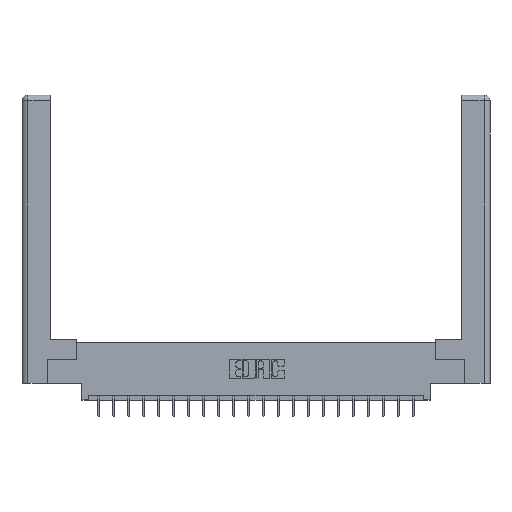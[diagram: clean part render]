
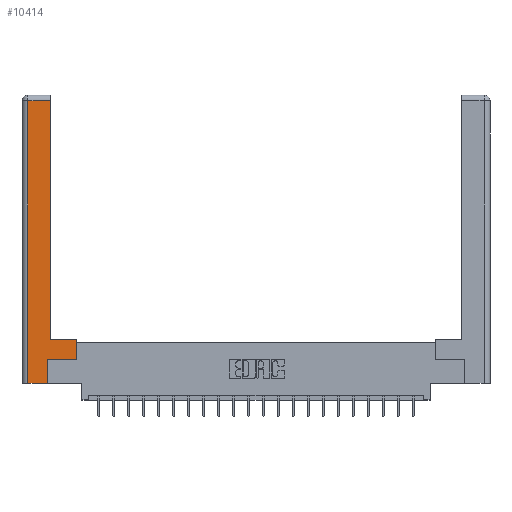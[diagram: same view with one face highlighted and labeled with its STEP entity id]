
A CAD part, top view. The second image highlights one B-rep face of the part: STEP entity #10414.
In plain terms, the highlighted planar face has unit normal (0, 0, 1).
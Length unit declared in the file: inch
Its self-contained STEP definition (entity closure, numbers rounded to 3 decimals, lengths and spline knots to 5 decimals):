
#24 = FACE_OUTER_BOUND ( 'NONE', #19741, .T. ) ;
#35 = LINE ( 'NONE', #14683, #7109 ) ;
#592 = CARTESIAN_POINT ( 'NONE',  ( 0.565, 0.245, 0. ) ) ;
#648 = DIRECTION ( 'NONE',  ( -1., 0., 0. ) ) ;
#887 = CARTESIAN_POINT ( 'NONE',  ( 0.0615, 2.94, 0. ) ) ;
#1226 = LINE ( 'NONE', #21098, #18644 ) ;
#1775 = VERTEX_POINT ( 'NONE', #4766 ) ;
#2141 = EDGE_CURVE ( 'NONE', #1775, #12506, #17856, .T. ) ;
#2516 = VECTOR ( 'NONE', #10026, 39.37008 ) ;
#2885 = EDGE_CURVE ( 'NONE', #7992, #18222, #19968, .T. ) ;
#3042 = EDGE_CURVE ( 'NONE', #20819, #6020, #1226, .T. ) ;
#4004 = DIRECTION ( 'NONE',  ( -1., 0., 0. ) ) ;
#4051 = CARTESIAN_POINT ( 'NONE',  ( 0.0615, 0., 0. ) ) ;
#4662 = AXIS2_PLACEMENT_3D ( 'NONE', #17757, #10466, #12505 ) ;
#4766 = CARTESIAN_POINT ( 'NONE',  ( 0.565, 0.45, 0. ) ) ;
#4906 = ORIENTED_EDGE ( 'NONE', *, *, #7469, .T. ) ;
#5986 = ORIENTED_EDGE ( 'NONE', *, *, #10708, .T. ) ;
#6020 = VERTEX_POINT ( 'NONE', #13642 ) ;
#6235 = ORIENTED_EDGE ( 'NONE', *, *, #14331, .T. ) ;
#6281 = VECTOR ( 'NONE', #20834, 39.37008 ) ;
#6994 = VERTEX_POINT ( 'NONE', #887 ) ;
#7109 = VECTOR ( 'NONE', #15374, 39.37008 ) ;
#7226 = VECTOR ( 'NONE', #4004, 39.37008 ) ;
#7335 = LINE ( 'NONE', #20233, #6281 ) ;
#7417 = CARTESIAN_POINT ( 'NONE',  ( 0.295, 0.45, 0. ) ) ;
#7469 = EDGE_CURVE ( 'NONE', #6994, #20819, #22369, .T. ) ;
#7992 = VERTEX_POINT ( 'NONE', #20230 ) ;
#8995 = ORIENTED_EDGE ( 'NONE', *, *, #2141, .T. ) ;
#10026 = DIRECTION ( 'NONE',  ( 0., -1., 0. ) ) ;
#10074 = ORIENTED_EDGE ( 'NONE', *, *, #3042, .T. ) ;
#10414 = ADVANCED_FACE ( 'NONE', ( #24 ), #10765, .F. ) ;
#10441 = VERTEX_POINT ( 'NONE', #19205 ) ;
#10466 = DIRECTION ( 'NONE',  ( 0., 0., -1. ) ) ;
#10708 = EDGE_CURVE ( 'NONE', #6020, #7992, #16348, .T. ) ;
#10765 = PLANE ( 'NONE',  #4662 ) ;
#10843 = EDGE_CURVE ( 'NONE', #12506, #10441, #7335, .T. ) ;
#11761 = DIRECTION ( 'NONE',  ( 1., 0., 0. ) ) ;
#11884 = VECTOR ( 'NONE', #648, 39.37008 ) ;
#12261 = VECTOR ( 'NONE', #18153, 39.37008 ) ;
#12505 = DIRECTION ( 'NONE',  ( -1., 0., 0. ) ) ;
#12506 = VERTEX_POINT ( 'NONE', #13411 ) ;
#13301 = CARTESIAN_POINT ( 'NONE',  ( 0.0615, 0., 0. ) ) ;
#13411 = CARTESIAN_POINT ( 'NONE',  ( 0.295, 0.45, 0. ) ) ;
#13642 = CARTESIAN_POINT ( 'NONE',  ( 0.265, 0., 0. ) ) ;
#14331 = EDGE_CURVE ( 'NONE', #18222, #1775, #35, .T. ) ;
#14551 = ORIENTED_EDGE ( 'NONE', *, *, #16783, .T. ) ;
#14683 = CARTESIAN_POINT ( 'NONE',  ( 0.565, 0.45, 0. ) ) ;
#15374 = DIRECTION ( 'NONE',  ( 0., 1., 0. ) ) ;
#16319 = DIRECTION ( 'NONE',  ( 1., 0., 0. ) ) ;
#16348 = LINE ( 'NONE', #21759, #12261 ) ;
#16439 = VECTOR ( 'NONE', #11761, 39.37008 ) ;
#16651 = ORIENTED_EDGE ( 'NONE', *, *, #2885, .T. ) ;
#16783 = EDGE_CURVE ( 'NONE', #10441, #6994, #17617, .T. ) ;
#17617 = LINE ( 'NONE', #21388, #11884 ) ;
#17757 = CARTESIAN_POINT ( 'NONE',  ( 0., 0., 0. ) ) ;
#17856 = LINE ( 'NONE', #7417, #7226 ) ;
#18153 = DIRECTION ( 'NONE',  ( 0., 1., 0. ) ) ;
#18164 = ORIENTED_EDGE ( 'NONE', *, *, #10843, .T. ) ;
#18222 = VERTEX_POINT ( 'NONE', #592 ) ;
#18644 = VECTOR ( 'NONE', #16319, 39.37008 ) ;
#19205 = CARTESIAN_POINT ( 'NONE',  ( 0.295, 2.94, 0. ) ) ;
#19741 = EDGE_LOOP ( 'NONE', ( #18164, #14551, #4906, #10074, #5986, #16651, #6235, #8995 ) ) ;
#19968 = LINE ( 'NONE', #20485, #16439 ) ;
#20230 = CARTESIAN_POINT ( 'NONE',  ( 0.265, 0.245, 0. ) ) ;
#20233 = CARTESIAN_POINT ( 'NONE',  ( 0.295, 3., 0. ) ) ;
#20485 = CARTESIAN_POINT ( 'NONE',  ( 0.565, 0.245, 0. ) ) ;
#20819 = VERTEX_POINT ( 'NONE', #4051 ) ;
#20834 = DIRECTION ( 'NONE',  ( 0., 1., 0. ) ) ;
#21098 = CARTESIAN_POINT ( 'NONE',  ( 0.265, 0., 0. ) ) ;
#21388 = CARTESIAN_POINT ( 'NONE',  ( 0.0615, 2.94, 0. ) ) ;
#21759 = CARTESIAN_POINT ( 'NONE',  ( 0.265, 0.245, 0. ) ) ;
#22369 = LINE ( 'NONE', #13301, #2516 ) ;
